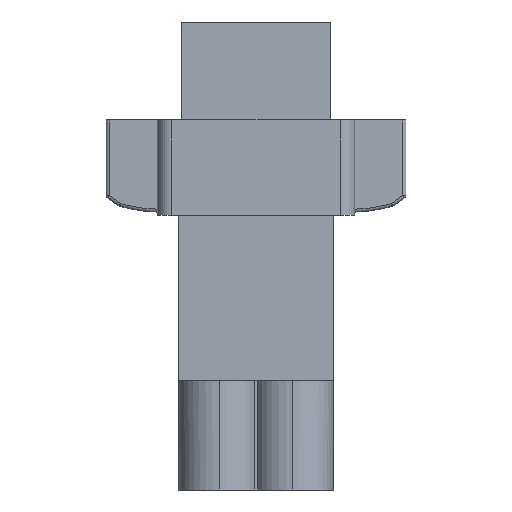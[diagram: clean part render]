
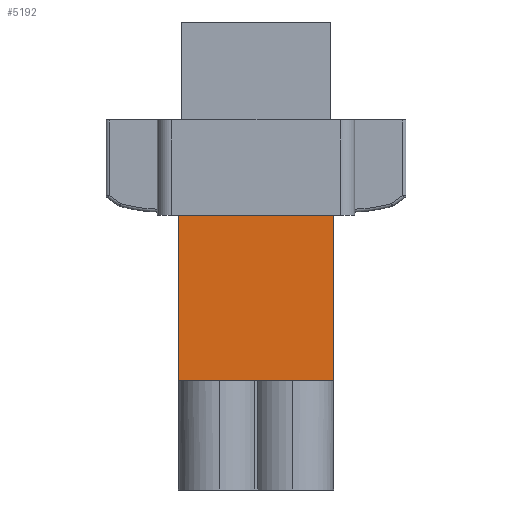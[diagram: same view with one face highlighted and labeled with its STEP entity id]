
A CAD part, front view. The second image highlights one B-rep face of the part: STEP entity #5192.
In plain terms, the highlighted planar face has unit normal (0, -1, 0).
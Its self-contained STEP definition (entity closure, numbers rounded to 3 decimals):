
#479 = EDGE_CURVE ( 'NONE', #7603, #11371, #2628, .T. ) ;
#711 = EDGE_CURVE ( 'NONE', #7603, #2415, #4489, .T. ) ;
#1265 = CARTESIAN_POINT ( 'NONE',  ( -2.5, -6.325, -11.3 ) ) ;
#1729 = EDGE_LOOP ( 'NONE', ( #3522, #4320, #9026, #10419 ) ) ;
#2403 = DIRECTION ( 'NONE',  ( 0., 0., 1. ) ) ;
#2415 = VERTEX_POINT ( 'NONE', #7050 ) ;
#2479 = CARTESIAN_POINT ( 'NONE',  ( 2.8, -6.325, 0. ) ) ;
#2628 = LINE ( 'NONE', #12237, #8600 ) ;
#2876 = CARTESIAN_POINT ( 'NONE',  ( 2.8, -6.325, -11.3 ) ) ;
#3522 = ORIENTED_EDGE ( 'NONE', *, *, #8465, .F. ) ;
#3618 = AXIS2_PLACEMENT_3D ( 'NONE', #1265, #10039, #5512 ) ;
#4320 = ORIENTED_EDGE ( 'NONE', *, *, #711, .F. ) ;
#4395 = CARTESIAN_POINT ( 'NONE',  ( 2.8, -6.325, -11.3 ) ) ;
#4489 = LINE ( 'NONE', #8608, #9804 ) ;
#4636 = VECTOR ( 'NONE', #8245, 1000. ) ;
#5192 = ADVANCED_FACE ( 'NONE', ( #6833 ), #8782, .T. ) ;
#5276 = CARTESIAN_POINT ( 'NONE',  ( -2.5, -6.325, 0. ) ) ;
#5512 = DIRECTION ( 'NONE',  ( 1., 0., 0. ) ) ;
#6074 = VERTEX_POINT ( 'NONE', #2479 ) ;
#6833 = FACE_OUTER_BOUND ( 'NONE', #1729, .T. ) ;
#7050 = CARTESIAN_POINT ( 'NONE',  ( -7.8, -6.325, 0. ) ) ;
#7603 = VERTEX_POINT ( 'NONE', #11040 ) ;
#8245 = DIRECTION ( 'NONE',  ( 0., 0., 1. ) ) ;
#8465 = EDGE_CURVE ( 'NONE', #2415, #6074, #11486, .T. ) ;
#8600 = VECTOR ( 'NONE', #10015, 1000. ) ;
#8608 = CARTESIAN_POINT ( 'NONE',  ( -7.8, -6.325, -11.3 ) ) ;
#8782 = PLANE ( 'NONE',  #3618 ) ;
#9026 = ORIENTED_EDGE ( 'NONE', *, *, #479, .T. ) ;
#9804 = VECTOR ( 'NONE', #2403, 1000. ) ;
#10015 = DIRECTION ( 'NONE',  ( 1., 0., 0. ) ) ;
#10039 = DIRECTION ( 'NONE',  ( 0., -1., 0. ) ) ;
#10127 = VECTOR ( 'NONE', #13372, 1000. ) ;
#10419 = ORIENTED_EDGE ( 'NONE', *, *, #13513, .T. ) ;
#11040 = CARTESIAN_POINT ( 'NONE',  ( -7.8, -6.325, -11.3 ) ) ;
#11371 = VERTEX_POINT ( 'NONE', #4395 ) ;
#11486 = LINE ( 'NONE', #5276, #10127 ) ;
#12237 = CARTESIAN_POINT ( 'NONE',  ( -2.5, -6.325, -11.3 ) ) ;
#12275 = LINE ( 'NONE', #2876, #4636 ) ;
#13372 = DIRECTION ( 'NONE',  ( 1., 0., 0. ) ) ;
#13513 = EDGE_CURVE ( 'NONE', #11371, #6074, #12275, .T. ) ;
